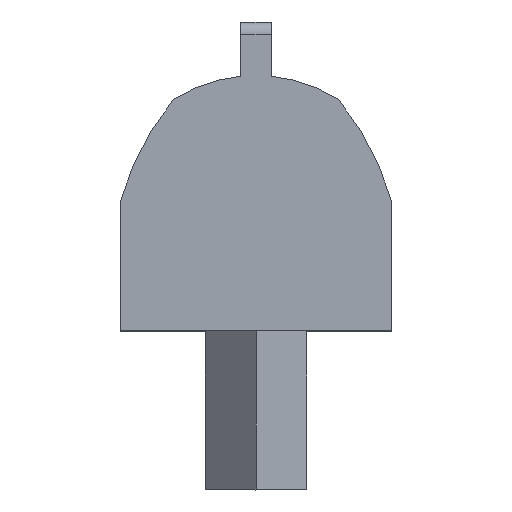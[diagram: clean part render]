
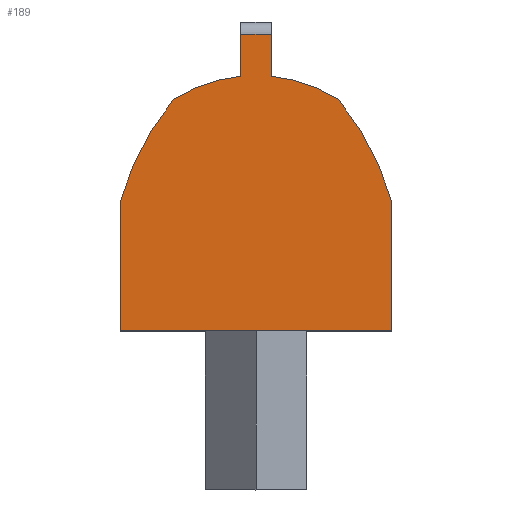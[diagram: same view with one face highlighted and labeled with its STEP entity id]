
A CAD part, top view. The second image highlights one B-rep face of the part: STEP entity #189.
In plain terms, the highlighted planar face has unit normal (0, 0, 1).
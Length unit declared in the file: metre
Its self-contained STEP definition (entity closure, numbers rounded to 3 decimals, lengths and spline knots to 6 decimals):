
#189 = ADVANCED_FACE( '', ( #442 ), #443, .T. );
#442 = FACE_OUTER_BOUND( '', #751, .T. );
#443 = PLANE( '', #752 );
#751 = EDGE_LOOP( '', ( #1335, #1336, #1337, #1338, #1339, #1340, #1341, #1342, #1343, #1344 ) );
#752 = AXIS2_PLACEMENT_3D( '', #1345, #1346, #1347 );
#1335 = ORIENTED_EDGE( '', *, *, #2175, .T. );
#1336 = ORIENTED_EDGE( '', *, *, #2176, .T. );
#1337 = ORIENTED_EDGE( '', *, *, #2177, .F. );
#1338 = ORIENTED_EDGE( '', *, *, #2178, .T. );
#1339 = ORIENTED_EDGE( '', *, *, #2164, .T. );
#1340 = ORIENTED_EDGE( '', *, *, #1968, .F. );
#1341 = ORIENTED_EDGE( '', *, *, #2179, .T. );
#1342 = ORIENTED_EDGE( '', *, *, #2126, .F. );
#1343 = ORIENTED_EDGE( '', *, *, #2180, .T. );
#1344 = ORIENTED_EDGE( '', *, *, #2181, .T. );
#1345 = CARTESIAN_POINT( '', ( 0., -0.003064, 0.15875 ) );
#1346 = DIRECTION( '', ( 0., 0., 1. ) );
#1347 = DIRECTION( '', ( 1., 0., 0. ) );
#1968 = EDGE_CURVE( '', #2376, #2365, #2378, .T. );
#2126 = EDGE_CURVE( '', #2647, #2649, #2650, .T. );
#2164 = EDGE_CURVE( '', #2706, #2365, #2707, .T. );
#2175 = EDGE_CURVE( '', #2721, #2722, #2723, .T. );
#2176 = EDGE_CURVE( '', #2722, #2724, #2725, .F. );
#2177 = EDGE_CURVE( '', #2726, #2724, #2727, .T. );
#2178 = EDGE_CURVE( '', #2726, #2706, #2728, .T. );
#2179 = EDGE_CURVE( '', #2376, #2649, #2729, .T. );
#2180 = EDGE_CURVE( '', #2647, #2730, #2731, .T. );
#2181 = EDGE_CURVE( '', #2730, #2721, #2732, .T. );
#2365 = VERTEX_POINT( '', #2966 );
#2376 = VERTEX_POINT( '', #2982 );
#2378 = LINE( '', #2985, #2986 );
#2647 = VERTEX_POINT( '', #3687 );
#2649 = VERTEX_POINT( '', #3690 );
#2650 = LINE( '', #3691, #3692 );
#2706 = VERTEX_POINT( '', #3777 );
#2707 = CIRCLE( '', #3778, 0.046958 );
#2721 = VERTEX_POINT( '', #3798 );
#2722 = VERTEX_POINT( '', #3799 );
#2723 = LINE( '', #3800, #3801 );
#2724 = VERTEX_POINT( '', #3802 );
#2725 = LINE( '', #3803, #3804 );
#2726 = VERTEX_POINT( '', #3805 );
#2727 = LINE( '', #3806, #3807 );
#2728 = CIRCLE( '', #3808, 0.025838 );
#2729 = LINE( '', #3809, #3810 );
#2730 = VERTEX_POINT( '', #3811 );
#2731 = CIRCLE( '', #3812, 0.046958 );
#2732 = CIRCLE( '', #3813, 0.025838 );
#2966 = CARTESIAN_POINT( '', ( -0.0225, -0.002757, 0.15875 ) );
#2982 = CARTESIAN_POINT( '', ( -0.0225, -0.024228, 0.15875 ) );
#2985 = CARTESIAN_POINT( '', ( -0.0225, -0.006178, 0.15875 ) );
#2986 = VECTOR( '', #4202, 1. );
#3687 = CARTESIAN_POINT( '', ( 0.0225, -0.002757, 0.15875 ) );
#3690 = CARTESIAN_POINT( '', ( 0.0225, -0.024228, 0.15875 ) );
#3691 = CARTESIAN_POINT( '', ( 0.0225, -0.006178, 0.15875 ) );
#3692 = VECTOR( '', #4353, 1. );
#3777 = CARTESIAN_POINT( '', ( -0.013584, 0.014241, 0.15875 ) );
#3778 = AXIS2_PLACEMENT_3D( '', #4389, #4390, #4391 );
#3798 = CARTESIAN_POINT( '', ( 0.0025, 0.017979, 0.15875 ) );
#3799 = CARTESIAN_POINT( '', ( 0.0025, 0.024979, 0.15875 ) );
#3800 = CARTESIAN_POINT( '', ( 0.0025, 0.022479, 0.15875 ) );
#3801 = VECTOR( '', #4404, 1. );
#3802 = CARTESIAN_POINT( '', ( -0.0025, 0.024979, 0.15875 ) );
#3803 = CARTESIAN_POINT( '', ( -0.0025, 0.024979, 0.15875 ) );
#3804 = VECTOR( '', #4405, 1. );
#3805 = CARTESIAN_POINT( '', ( -0.0025, 0.017979, 0.15875 ) );
#3806 = CARTESIAN_POINT( '', ( -0.0025, 0.022479, 0.15875 ) );
#3807 = VECTOR( '', #4406, 1. );
#3808 = AXIS2_PLACEMENT_3D( '', #4407, #4408, #4409 );
#3809 = CARTESIAN_POINT( '', ( 0., -0.024228, 0.15875 ) );
#3810 = VECTOR( '', #4410, 1. );
#3811 = CARTESIAN_POINT( '', ( 0.013584, 0.014241, 0.15875 ) );
#3812 = AXIS2_PLACEMENT_3D( '', #4411, #4412, #4413 );
#3813 = AXIS2_PLACEMENT_3D( '', #4414, #4415, #4416 );
#4202 = DIRECTION( '', ( 0., 1., 0. ) );
#4353 = DIRECTION( '', ( 0., -1., 0. ) );
#4389 = CARTESIAN_POINT( '', ( 0.022665, -0.01561, 0.15875 ) );
#4390 = DIRECTION( '', ( 0., 0., 1. ) );
#4391 = DIRECTION( '', ( 1., 0., 0. ) );
#4404 = DIRECTION( '', ( 0., 1., 0. ) );
#4405 = DIRECTION( '', ( 1., 0., 0. ) );
#4406 = DIRECTION( '', ( 0., 1., 0. ) );
#4407 = CARTESIAN_POINT( '', ( 0., -0.007738, 0.15875 ) );
#4408 = DIRECTION( '', ( 0., 0., 1. ) );
#4409 = DIRECTION( '', ( 1., 0., 0. ) );
#4410 = DIRECTION( '', ( 1., 0., 0. ) );
#4411 = CARTESIAN_POINT( '', ( -0.022665, -0.01561, 0.15875 ) );
#4412 = DIRECTION( '', ( 0., 0., 1. ) );
#4413 = DIRECTION( '', ( 1., 0., 0. ) );
#4414 = CARTESIAN_POINT( '', ( 0., -0.007738, 0.15875 ) );
#4415 = DIRECTION( '', ( 0., 0., 1. ) );
#4416 = DIRECTION( '', ( 1., 0., 0. ) );
